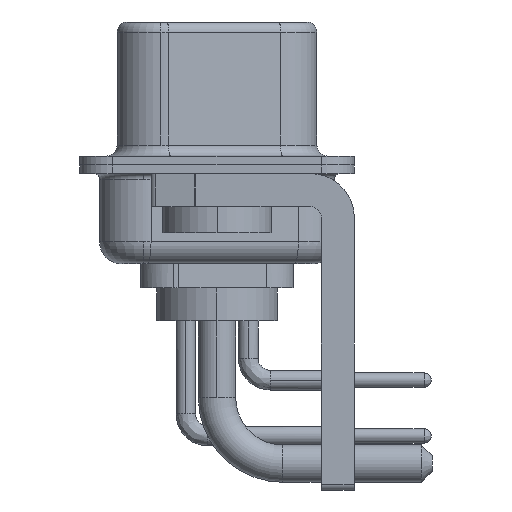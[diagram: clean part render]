
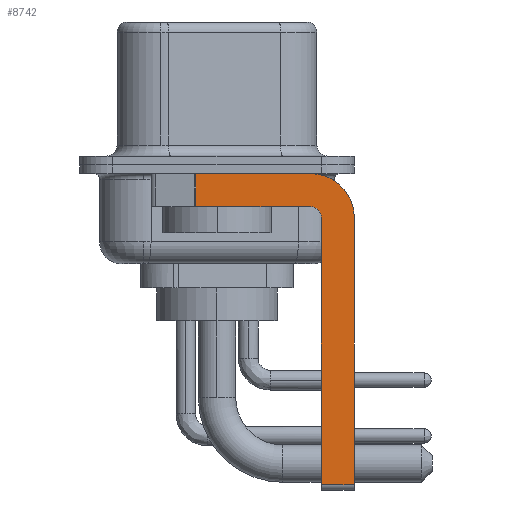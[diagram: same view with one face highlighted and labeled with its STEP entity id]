
A CAD part, left-side view. The second image highlights one B-rep face of the part: STEP entity #8742.
In plain terms, the highlighted planar face has unit normal (-1, 0, 0).
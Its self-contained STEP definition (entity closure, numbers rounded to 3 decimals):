
#427 = LINE ( 'NONE', #22681, #10363 ) ;
#899 = CARTESIAN_POINT ( 'NONE',  ( -2.9, -4.75, -14.55 ) ) ;
#1016 = CARTESIAN_POINT ( 'NONE',  ( -2.9, -4.75, -2.4 ) ) ;
#1254 = LINE ( 'NONE', #22014, #11170 ) ;
#1554 = DIRECTION ( 'NONE',  ( 0., -1., 0. ) ) ;
#2513 = VERTEX_POINT ( 'NONE', #899 ) ;
#2582 = VERTEX_POINT ( 'NONE', #28334 ) ;
#2937 = VERTEX_POINT ( 'NONE', #24275 ) ;
#4248 = CARTESIAN_POINT ( 'NONE',  ( -2.9, -4.25, -2.4 ) ) ;
#4520 = VECTOR ( 'NONE', #27336, 1000. ) ;
#4647 = ORIENTED_EDGE ( 'NONE', *, *, #18684, .F. ) ;
#4652 = AXIS2_PLACEMENT_3D ( 'NONE', #19681, #25016, #13804 ) ;
#4860 = CARTESIAN_POINT ( 'NONE',  ( -2.9, 0.978, -0.4 ) ) ;
#6325 = CARTESIAN_POINT ( 'NONE',  ( -2.9, -4.25, -2.4 ) ) ;
#6379 = LINE ( 'NONE', #29336, #6719 ) ;
#6719 = VECTOR ( 'NONE', #24609, 1000. ) ;
#6788 = ORIENTED_EDGE ( 'NONE', *, *, #14027, .T. ) ;
#7531 = CARTESIAN_POINT ( 'NONE',  ( -2.9, 0.978, -1.9 ) ) ;
#8707 = DIRECTION ( 'NONE',  ( 1., 0., 0. ) ) ;
#8742 = ADVANCED_FACE ( 'NONE', ( #24849 ), #10810, .F. ) ;
#9913 = ORIENTED_EDGE ( 'NONE', *, *, #17327, .F. ) ;
#10147 = AXIS2_PLACEMENT_3D ( 'NONE', #4248, #11117, #13365 ) ;
#10363 = VECTOR ( 'NONE', #11611, 1000. ) ;
#10501 = EDGE_LOOP ( 'NONE', ( #21446, #6788, #24105, #17790, #15934, #20303, #4647, #9913 ) ) ;
#10686 = VERTEX_POINT ( 'NONE', #28271 ) ;
#10810 = PLANE ( 'NONE',  #17544 ) ;
#11117 = DIRECTION ( 'NONE',  ( 1., 0., 0. ) ) ;
#11170 = VECTOR ( 'NONE', #1554, 1000. ) ;
#11174 = EDGE_CURVE ( 'NONE', #15192, #12866, #427, .T. ) ;
#11484 = VERTEX_POINT ( 'NONE', #1016 ) ;
#11611 = DIRECTION ( 'NONE',  ( 0., -1., 0. ) ) ;
#12712 = VERTEX_POINT ( 'NONE', #23357 ) ;
#12866 = VERTEX_POINT ( 'NONE', #15537 ) ;
#13251 = CIRCLE ( 'NONE', #4652, 0.5 ) ;
#13365 = DIRECTION ( 'NONE',  ( 0., 0., -1. ) ) ;
#13804 = DIRECTION ( 'NONE',  ( 0., 0., 1. ) ) ;
#14027 = EDGE_CURVE ( 'NONE', #15192, #10686, #28409, .T. ) ;
#14078 = LINE ( 'NONE', #27960, #28327 ) ;
#14847 = DIRECTION ( 'NONE',  ( 0., 0., -1. ) ) ;
#15192 = VERTEX_POINT ( 'NONE', #4860 ) ;
#15426 = CIRCLE ( 'NONE', #10147, 2. ) ;
#15537 = CARTESIAN_POINT ( 'NONE',  ( -2.9, -4.25, -0.4 ) ) ;
#15934 = ORIENTED_EDGE ( 'NONE', *, *, #18965, .F. ) ;
#17327 = EDGE_CURVE ( 'NONE', #12866, #2937, #15426, .T. ) ;
#17544 = AXIS2_PLACEMENT_3D ( 'NONE', #6325, #8707, #17717 ) ;
#17717 = DIRECTION ( 'NONE',  ( 0., 0., -1. ) ) ;
#17790 = ORIENTED_EDGE ( 'NONE', *, *, #21456, .F. ) ;
#18684 = EDGE_CURVE ( 'NONE', #2937, #12712, #14078, .T. ) ;
#18764 = EDGE_CURVE ( 'NONE', #2513, #12712, #1254, .T. ) ;
#18965 = EDGE_CURVE ( 'NONE', #2513, #11484, #20509, .T. ) ;
#19681 = CARTESIAN_POINT ( 'NONE',  ( -2.9, -4.25, -2.4 ) ) ;
#20303 = ORIENTED_EDGE ( 'NONE', *, *, #18764, .T. ) ;
#20509 = LINE ( 'NONE', #27060, #4520 ) ;
#21427 = DIRECTION ( 'NONE',  ( 0., 0., -1. ) ) ;
#21446 = ORIENTED_EDGE ( 'NONE', *, *, #11174, .F. ) ;
#21456 = EDGE_CURVE ( 'NONE', #11484, #2582, #13251, .T. ) ;
#22014 = CARTESIAN_POINT ( 'NONE',  ( -2.9, -4.25, -14.55 ) ) ;
#22681 = CARTESIAN_POINT ( 'NONE',  ( -2.9, 3., -0.4 ) ) ;
#23357 = CARTESIAN_POINT ( 'NONE',  ( -2.9, -6.25, -14.55 ) ) ;
#24105 = ORIENTED_EDGE ( 'NONE', *, *, #26359, .F. ) ;
#24275 = CARTESIAN_POINT ( 'NONE',  ( -2.9, -6.25, -2.4 ) ) ;
#24609 = DIRECTION ( 'NONE',  ( 0., 1., 0. ) ) ;
#24849 = FACE_OUTER_BOUND ( 'NONE', #10501, .T. ) ;
#25016 = DIRECTION ( 'NONE',  ( -1., 0., 0. ) ) ;
#26359 = EDGE_CURVE ( 'NONE', #2582, #10686, #6379, .T. ) ;
#27060 = CARTESIAN_POINT ( 'NONE',  ( -2.9, -4.75, -14.8 ) ) ;
#27336 = DIRECTION ( 'NONE',  ( 0., 0., 1. ) ) ;
#27960 = CARTESIAN_POINT ( 'NONE',  ( -2.9, -6.25, -2.4 ) ) ;
#28125 = VECTOR ( 'NONE', #14847, 1000. ) ;
#28271 = CARTESIAN_POINT ( 'NONE',  ( -2.9, 0.978, -1.9 ) ) ;
#28327 = VECTOR ( 'NONE', #21427, 1000. ) ;
#28334 = CARTESIAN_POINT ( 'NONE',  ( -2.9, -4.25, -1.9 ) ) ;
#28409 = LINE ( 'NONE', #7531, #28125 ) ;
#29336 = CARTESIAN_POINT ( 'NONE',  ( -2.9, -4.25, -1.9 ) ) ;
